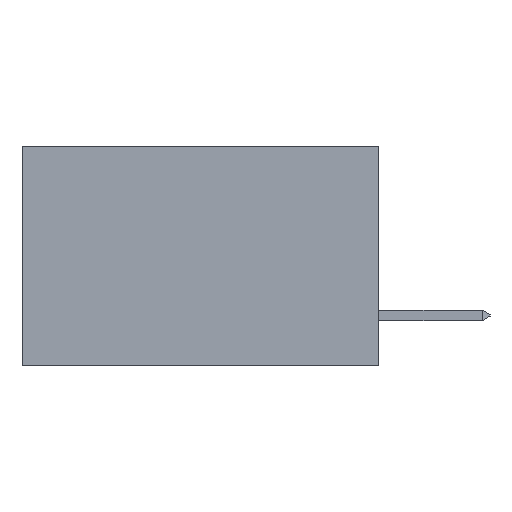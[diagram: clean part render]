
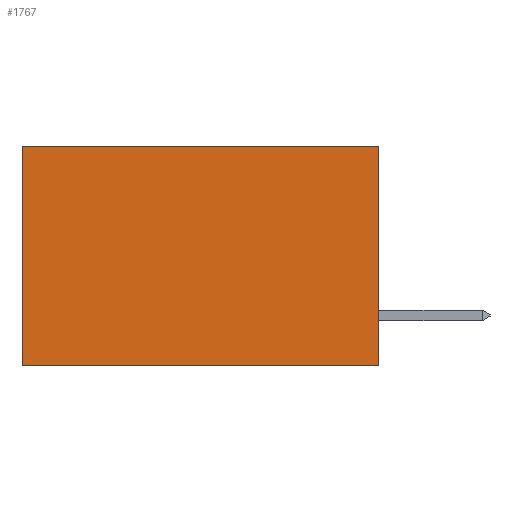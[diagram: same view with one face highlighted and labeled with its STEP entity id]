
A CAD part, left-side view. The second image highlights one B-rep face of the part: STEP entity #1767.
In plain terms, the highlighted planar face has unit normal (-1, 0, 0).
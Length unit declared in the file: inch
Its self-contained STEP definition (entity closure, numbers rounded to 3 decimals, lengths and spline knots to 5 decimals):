
#183 = ORIENTED_EDGE ( 'NONE', *, *, #5081, .F. ) ;
#377 = VERTEX_POINT ( 'NONE', #4501 ) ;
#482 = EDGE_LOOP ( 'NONE', ( #1006, #730, #183, #8540 ) ) ;
#730 = ORIENTED_EDGE ( 'NONE', *, *, #1910, .F. ) ;
#1006 = ORIENTED_EDGE ( 'NONE', *, *, #2406, .T. ) ;
#1767 = ADVANCED_FACE ( 'NONE', ( #9099 ), #9200, .F. ) ;
#1910 = EDGE_CURVE ( 'NONE', #3409, #2430, #7558, .T. ) ;
#2338 = VERTEX_POINT ( 'NONE', #3538 ) ;
#2406 = EDGE_CURVE ( 'NONE', #2338, #2430, #2918, .T. ) ;
#2430 = VERTEX_POINT ( 'NONE', #3583 ) ;
#2744 = LINE ( 'NONE', #5033, #6881 ) ;
#2918 = LINE ( 'NONE', #9231, #7043 ) ;
#3409 = VERTEX_POINT ( 'NONE', #8726 ) ;
#3473 = DIRECTION ( 'NONE',  ( 0., 0., -1. ) ) ;
#3538 = CARTESIAN_POINT ( 'NONE',  ( 0.298, 0.6, 0. ) ) ;
#3583 = CARTESIAN_POINT ( 'NONE',  ( 0.298, 0.6, -0.37 ) ) ;
#4139 = DIRECTION ( 'NONE',  ( 0., 0., -1. ) ) ;
#4383 = DIRECTION ( 'NONE',  ( 0., 1., 0. ) ) ;
#4501 = CARTESIAN_POINT ( 'NONE',  ( 0.298, 0., 0. ) ) ;
#4660 = DIRECTION ( 'NONE',  ( 0., 0., -1. ) ) ;
#5033 = CARTESIAN_POINT ( 'NONE',  ( 0.298, 0., 0. ) ) ;
#5081 = EDGE_CURVE ( 'NONE', #377, #3409, #7757, .T. ) ;
#5422 = DIRECTION ( 'NONE',  ( 1., 0., 0. ) ) ;
#5662 = VECTOR ( 'NONE', #4383, 39.37008 ) ;
#6046 = CARTESIAN_POINT ( 'NONE',  ( 0.298, 0., -0.37 ) ) ;
#6656 = DIRECTION ( 'NONE',  ( 0., 1., 0. ) ) ;
#6881 = VECTOR ( 'NONE', #6656, 39.37008 ) ;
#7043 = VECTOR ( 'NONE', #3473, 39.37008 ) ;
#7558 = LINE ( 'NONE', #6046, #5662 ) ;
#7757 = LINE ( 'NONE', #8265, #9429 ) ;
#8265 = CARTESIAN_POINT ( 'NONE',  ( 0.298, 0., 0. ) ) ;
#8473 = AXIS2_PLACEMENT_3D ( 'NONE', #10655, #5422, #4660 ) ;
#8540 = ORIENTED_EDGE ( 'NONE', *, *, #9443, .T. ) ;
#8726 = CARTESIAN_POINT ( 'NONE',  ( 0.298, 0., -0.37 ) ) ;
#9099 = FACE_OUTER_BOUND ( 'NONE', #482, .T. ) ;
#9200 = PLANE ( 'NONE',  #8473 ) ;
#9231 = CARTESIAN_POINT ( 'NONE',  ( 0.298, 0.6, 0. ) ) ;
#9429 = VECTOR ( 'NONE', #4139, 39.37008 ) ;
#9443 = EDGE_CURVE ( 'NONE', #377, #2338, #2744, .T. ) ;
#10655 = CARTESIAN_POINT ( 'NONE',  ( 0.298, 0., 0. ) ) ;
